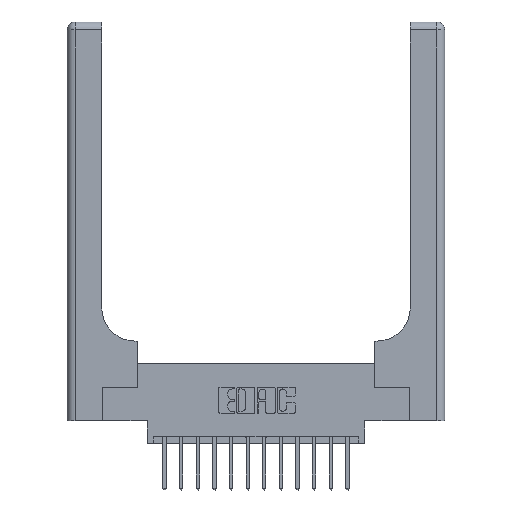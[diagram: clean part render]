
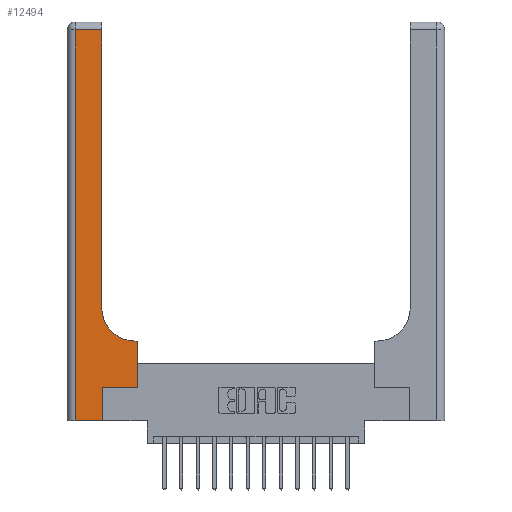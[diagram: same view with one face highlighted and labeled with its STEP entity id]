
A CAD part, top view. The second image highlights one B-rep face of the part: STEP entity #12494.
In plain terms, the highlighted planar face has unit normal (0, 0, 1).
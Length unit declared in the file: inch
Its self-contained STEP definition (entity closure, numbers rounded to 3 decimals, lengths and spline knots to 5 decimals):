
#173 = CARTESIAN_POINT ( 'NONE',  ( 0.06, 3., 0.37 ) ) ;
#202 = DIRECTION ( 'NONE',  ( 0., 0., -1. ) ) ;
#204 = CARTESIAN_POINT ( 'NONE',  ( 0.26, 0.6, 0.37 ) ) ;
#383 = EDGE_CURVE ( 'NONE', #6574, #11732, #6160, .T. ) ;
#575 = VERTEX_POINT ( 'NONE', #5872 ) ;
#643 = VERTEX_POINT ( 'NONE', #14669 ) ;
#745 = VECTOR ( 'NONE', #17294, 39.37008 ) ;
#875 = CARTESIAN_POINT ( 'NONE',  ( 0., 2.94, 0.37 ) ) ;
#1160 = VECTOR ( 'NONE', #5572, 39.37008 ) ;
#1547 = CARTESIAN_POINT ( 'NONE',  ( 0.51, 0.85, 0.37 ) ) ;
#2206 = LINE ( 'NONE', #875, #8140 ) ;
#2323 = VECTOR ( 'NONE', #5906, 39.37008 ) ;
#2557 = AXIS2_PLACEMENT_3D ( 'NONE', #7259, #12590, #3389 ) ;
#3099 = CARTESIAN_POINT ( 'NONE',  ( 0.265, 0.25, 0.37 ) ) ;
#3204 = CARTESIAN_POINT ( 'NONE',  ( 0.26, 0.85, 0.37 ) ) ;
#3389 = DIRECTION ( 'NONE',  ( -1., 0., 0. ) ) ;
#3827 = EDGE_CURVE ( 'NONE', #16842, #4128, #4357, .T. ) ;
#4128 = VERTEX_POINT ( 'NONE', #17054 ) ;
#4141 = CARTESIAN_POINT ( 'NONE',  ( 0.51, 0.6, 0.37 ) ) ;
#4280 = CARTESIAN_POINT ( 'NONE',  ( 0.26, 3., 0.37 ) ) ;
#4357 = LINE ( 'NONE', #4280, #1160 ) ;
#4383 = PLANE ( 'NONE',  #2557 ) ;
#4543 = VECTOR ( 'NONE', #16432, 39.37008 ) ;
#5350 = AXIS2_PLACEMENT_3D ( 'NONE', #1547, #202, #12359 ) ;
#5572 = DIRECTION ( 'NONE',  ( 0., 1., 0. ) ) ;
#5872 = CARTESIAN_POINT ( 'NONE',  ( 0.528, 0.6, 0.37 ) ) ;
#5906 = DIRECTION ( 'NONE',  ( 1., 0., 0. ) ) ;
#6160 = LINE ( 'NONE', #11630, #2323 ) ;
#6293 = DIRECTION ( 'NONE',  ( -1., 0., 0. ) ) ;
#6376 = CARTESIAN_POINT ( 'NONE',  ( 0., 0., 0.37 ) ) ;
#6574 = VERTEX_POINT ( 'NONE', #3099 ) ;
#6737 = LINE ( 'NONE', #173, #10289 ) ;
#7021 = LINE ( 'NONE', #16528, #4543 ) ;
#7259 = CARTESIAN_POINT ( 'NONE',  ( 0., 3., 0.37 ) ) ;
#8140 = VECTOR ( 'NONE', #6293, 39.37008 ) ;
#8562 = FACE_OUTER_BOUND ( 'NONE', #13563, .T. ) ;
#8582 = CARTESIAN_POINT ( 'NONE',  ( 0.265, 0., 0.37 ) ) ;
#8850 = ORIENTED_EDGE ( 'NONE', *, *, #9032, .T. ) ;
#9032 = EDGE_CURVE ( 'NONE', #575, #14519, #12361, .T. ) ;
#9116 = VERTEX_POINT ( 'NONE', #8582 ) ;
#9782 = DIRECTION ( 'NONE',  ( -1., 0., 0. ) ) ;
#9816 = EDGE_CURVE ( 'NONE', #9116, #6574, #15967, .T. ) ;
#10289 = VECTOR ( 'NONE', #12238, 39.37008 ) ;
#10340 = DIRECTION ( 'NONE',  ( 0., 1., 0. ) ) ;
#10940 = ORIENTED_EDGE ( 'NONE', *, *, #16272, .T. ) ;
#11023 = VERTEX_POINT ( 'NONE', #12319 ) ;
#11052 = ORIENTED_EDGE ( 'NONE', *, *, #11887, .T. ) ;
#11178 = ORIENTED_EDGE ( 'NONE', *, *, #3827, .T. ) ;
#11630 = CARTESIAN_POINT ( 'NONE',  ( 0.265, 0.25, 0.37 ) ) ;
#11732 = VERTEX_POINT ( 'NONE', #17161 ) ;
#11887 = EDGE_CURVE ( 'NONE', #14519, #16842, #16756, .T. ) ;
#12238 = DIRECTION ( 'NONE',  ( 0., -1., 0. ) ) ;
#12319 = CARTESIAN_POINT ( 'NONE',  ( 0.06, 0., 0.37 ) ) ;
#12359 = DIRECTION ( 'NONE',  ( 1., 0., 0. ) ) ;
#12361 = LINE ( 'NONE', #204, #15611 ) ;
#12494 = ADVANCED_FACE ( 'NONE', ( #8562 ), #4383, .F. ) ;
#12590 = DIRECTION ( 'NONE',  ( 0., 0., -1. ) ) ;
#12656 = EDGE_CURVE ( 'NONE', #4128, #643, #2206, .T. ) ;
#12965 = ORIENTED_EDGE ( 'NONE', *, *, #13538, .T. ) ;
#13173 = LINE ( 'NONE', #6376, #745 ) ;
#13538 = EDGE_CURVE ( 'NONE', #11732, #575, #7021, .T. ) ;
#13563 = EDGE_LOOP ( 'NONE', ( #11178, #15744, #10940, #16916, #17296, #15406, #12965, #8850, #11052 ) ) ;
#14519 = VERTEX_POINT ( 'NONE', #4141 ) ;
#14669 = CARTESIAN_POINT ( 'NONE',  ( 0.06, 2.94, 0.37 ) ) ;
#14843 = EDGE_CURVE ( 'NONE', #11023, #9116, #13173, .T. ) ;
#15406 = ORIENTED_EDGE ( 'NONE', *, *, #383, .T. ) ;
#15611 = VECTOR ( 'NONE', #9782, 39.37008 ) ;
#15744 = ORIENTED_EDGE ( 'NONE', *, *, #12656, .T. ) ;
#15933 = VECTOR ( 'NONE', #10340, 39.37008 ) ;
#15967 = LINE ( 'NONE', #17022, #15933 ) ;
#16272 = EDGE_CURVE ( 'NONE', #643, #11023, #6737, .T. ) ;
#16432 = DIRECTION ( 'NONE',  ( 0., 1., 0. ) ) ;
#16528 = CARTESIAN_POINT ( 'NONE',  ( 0.528, 0.25, 0.37 ) ) ;
#16756 = CIRCLE ( 'NONE', #5350, 0.25 ) ;
#16842 = VERTEX_POINT ( 'NONE', #3204 ) ;
#16916 = ORIENTED_EDGE ( 'NONE', *, *, #14843, .T. ) ;
#17022 = CARTESIAN_POINT ( 'NONE',  ( 0.265, 0., 0.37 ) ) ;
#17054 = CARTESIAN_POINT ( 'NONE',  ( 0.26, 2.94, 0.37 ) ) ;
#17161 = CARTESIAN_POINT ( 'NONE',  ( 0.528, 0.25, 0.37 ) ) ;
#17294 = DIRECTION ( 'NONE',  ( 1., 0., 0. ) ) ;
#17296 = ORIENTED_EDGE ( 'NONE', *, *, #9816, .T. ) ;
